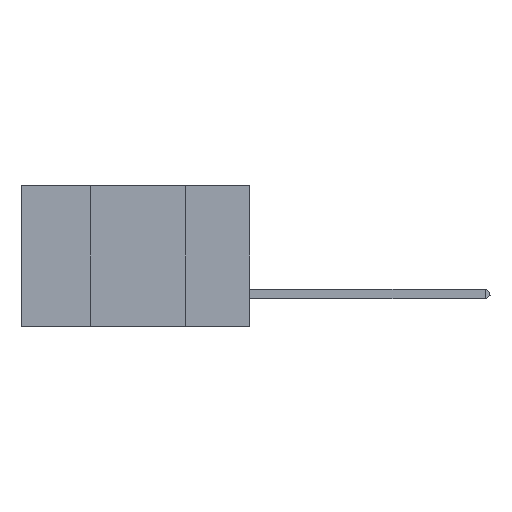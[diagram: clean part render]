
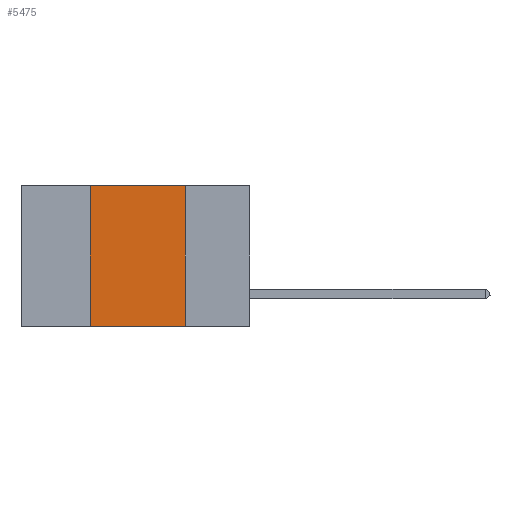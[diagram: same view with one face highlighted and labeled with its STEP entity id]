
A CAD part, left-side view. The second image highlights one B-rep face of the part: STEP entity #5475.
In plain terms, the highlighted planar face has unit normal (-1, 0, 0).
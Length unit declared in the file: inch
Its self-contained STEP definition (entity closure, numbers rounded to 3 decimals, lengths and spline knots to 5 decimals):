
#78 = FACE_OUTER_BOUND ( 'NONE', #1066, .T. ) ;
#384 = CARTESIAN_POINT ( 'NONE',  ( 0., 0.17, 0. ) ) ;
#1066 = EDGE_LOOP ( 'NONE', ( #7381, #17036, #14636, #17782 ) ) ;
#1071 = EDGE_CURVE ( 'NONE', #8507, #10897, #10795, .T. ) ;
#1338 = AXIS2_PLACEMENT_3D ( 'NONE', #15012, #9738, #19750 ) ;
#1648 = DIRECTION ( 'NONE',  ( 0., -1., 0. ) ) ;
#3219 = DIRECTION ( 'NONE',  ( 0., -1., 0. ) ) ;
#3425 = VECTOR ( 'NONE', #1648, 39.37008 ) ;
#5394 = VERTEX_POINT ( 'NONE', #11461 ) ;
#5475 = ADVANCED_FACE ( 'NONE', ( #78 ), #8149, .F. ) ;
#6596 = VECTOR ( 'NONE', #3219, 39.37008 ) ;
#6834 = DIRECTION ( 'NONE',  ( 0., 0., -1. ) ) ;
#7381 = ORIENTED_EDGE ( 'NONE', *, *, #19249, .F. ) ;
#8149 = PLANE ( 'NONE',  #1338 ) ;
#8507 = VERTEX_POINT ( 'NONE', #21232 ) ;
#9360 = LINE ( 'NONE', #384, #14873 ) ;
#9738 = DIRECTION ( 'NONE',  ( 1., 0., 0. ) ) ;
#9817 = CARTESIAN_POINT ( 'NONE',  ( 0., 0.17, -0.37 ) ) ;
#10748 = EDGE_CURVE ( 'NONE', #10897, #5394, #11161, .T. ) ;
#10795 = LINE ( 'NONE', #19003, #13932 ) ;
#10897 = VERTEX_POINT ( 'NONE', #17650 ) ;
#11161 = LINE ( 'NONE', #19699, #3425 ) ;
#11461 = CARTESIAN_POINT ( 'NONE',  ( 0., 0.17, 0. ) ) ;
#13932 = VECTOR ( 'NONE', #15892, 39.37008 ) ;
#14636 = ORIENTED_EDGE ( 'NONE', *, *, #1071, .F. ) ;
#14873 = VECTOR ( 'NONE', #6834, 39.37008 ) ;
#15012 = CARTESIAN_POINT ( 'NONE',  ( 0., 0.6, 0. ) ) ;
#15892 = DIRECTION ( 'NONE',  ( 0., 0., 1. ) ) ;
#16558 = CARTESIAN_POINT ( 'NONE',  ( 0., 0.6, -0.37 ) ) ;
#17036 = ORIENTED_EDGE ( 'NONE', *, *, #10748, .F. ) ;
#17650 = CARTESIAN_POINT ( 'NONE',  ( 0., 0.42, 0. ) ) ;
#17782 = ORIENTED_EDGE ( 'NONE', *, *, #21012, .T. ) ;
#19003 = CARTESIAN_POINT ( 'NONE',  ( 0., 0.42, 0. ) ) ;
#19249 = EDGE_CURVE ( 'NONE', #5394, #19781, #9360, .T. ) ;
#19699 = CARTESIAN_POINT ( 'NONE',  ( 0., 0.6, 0. ) ) ;
#19750 = DIRECTION ( 'NONE',  ( 0., 0., -1. ) ) ;
#19781 = VERTEX_POINT ( 'NONE', #9817 ) ;
#19955 = LINE ( 'NONE', #16558, #6596 ) ;
#21012 = EDGE_CURVE ( 'NONE', #8507, #19781, #19955, .T. ) ;
#21232 = CARTESIAN_POINT ( 'NONE',  ( 0., 0.42, -0.37 ) ) ;
